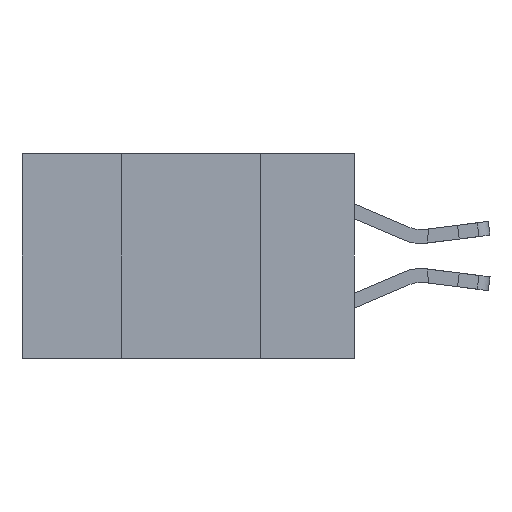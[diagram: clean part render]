
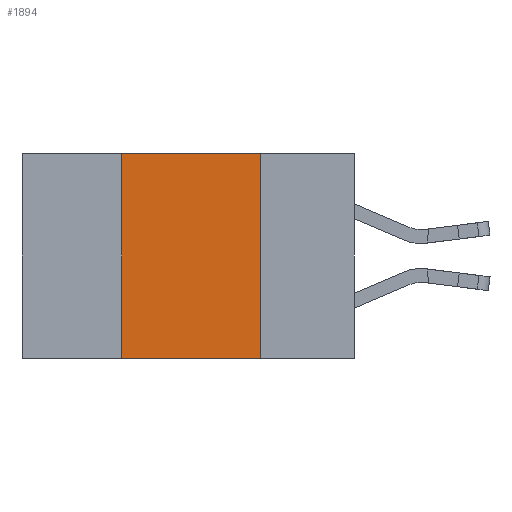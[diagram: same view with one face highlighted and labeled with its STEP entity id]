
A CAD part, left-side view. The second image highlights one B-rep face of the part: STEP entity #1894.
In plain terms, the highlighted planar face has unit normal (-1, 0, 0).
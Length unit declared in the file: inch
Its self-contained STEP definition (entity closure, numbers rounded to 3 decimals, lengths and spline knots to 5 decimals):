
#19 = DIRECTION ( 'NONE',  ( 0., -1., 0. ) ) ;
#142 = CARTESIAN_POINT ( 'NONE',  ( 0., 0.17, -0.37 ) ) ;
#205 = CARTESIAN_POINT ( 'NONE',  ( 0., 0.6, 0. ) ) ;
#536 = CARTESIAN_POINT ( 'NONE',  ( 0., 0.17, -0.37 ) ) ;
#946 = DIRECTION ( 'NONE',  ( 0., 0., -1. ) ) ;
#1259 = DIRECTION ( 'NONE',  ( 0., 0., -1. ) ) ;
#1294 = DIRECTION ( 'NONE',  ( 1., 0., 0. ) ) ;
#1385 = AXIS2_PLACEMENT_3D ( 'NONE', #1695, #1294, #1259 ) ;
#1695 = CARTESIAN_POINT ( 'NONE',  ( 0., 0.6, 0. ) ) ;
#1894 = ADVANCED_FACE ( 'NONE', ( #11767 ), #2211, .F. ) ;
#1951 = ORIENTED_EDGE ( 'NONE', *, *, #11916, .F. ) ;
#2211 = PLANE ( 'NONE',  #1385 ) ;
#2762 = VECTOR ( 'NONE', #7701, 39.37008 ) ;
#5325 = ORIENTED_EDGE ( 'NONE', *, *, #11917, .F. ) ;
#5701 = ORIENTED_EDGE ( 'NONE', *, *, #12591, .T. ) ;
#6275 = LINE ( 'NONE', #12785, #12216 ) ;
#6808 = CARTESIAN_POINT ( 'NONE',  ( 0., 0.17, 0. ) ) ;
#7701 = DIRECTION ( 'NONE',  ( 0., -1., 0. ) ) ;
#7784 = VECTOR ( 'NONE', #19, 39.37008 ) ;
#7933 = CARTESIAN_POINT ( 'NONE',  ( 0., 0.6, -0.37 ) ) ;
#8031 = VERTEX_POINT ( 'NONE', #6808 ) ;
#8156 = LINE ( 'NONE', #205, #7784 ) ;
#8536 = ORIENTED_EDGE ( 'NONE', *, *, #12148, .F. ) ;
#9652 = LINE ( 'NONE', #7933, #2762 ) ;
#9875 = VERTEX_POINT ( 'NONE', #13722 ) ;
#11354 = VERTEX_POINT ( 'NONE', #142 ) ;
#11767 = FACE_OUTER_BOUND ( 'NONE', #14696, .T. ) ;
#11916 = EDGE_CURVE ( 'NONE', #8031, #11354, #14149, .T. ) ;
#11917 = EDGE_CURVE ( 'NONE', #13762, #8031, #8156, .T. ) ;
#12148 = EDGE_CURVE ( 'NONE', #9875, #13762, #6275, .T. ) ;
#12216 = VECTOR ( 'NONE', #12724, 39.37008 ) ;
#12591 = EDGE_CURVE ( 'NONE', #9875, #11354, #9652, .T. ) ;
#12646 = CARTESIAN_POINT ( 'NONE',  ( 0., 0.42, 0. ) ) ;
#12724 = DIRECTION ( 'NONE',  ( 0., 0., 1. ) ) ;
#12785 = CARTESIAN_POINT ( 'NONE',  ( 0., 0.42, -0.37 ) ) ;
#13722 = CARTESIAN_POINT ( 'NONE',  ( 0., 0.42, -0.37 ) ) ;
#13762 = VERTEX_POINT ( 'NONE', #12646 ) ;
#13853 = VECTOR ( 'NONE', #946, 39.37008 ) ;
#14149 = LINE ( 'NONE', #536, #13853 ) ;
#14696 = EDGE_LOOP ( 'NONE', ( #1951, #5325, #8536, #5701 ) ) ;
